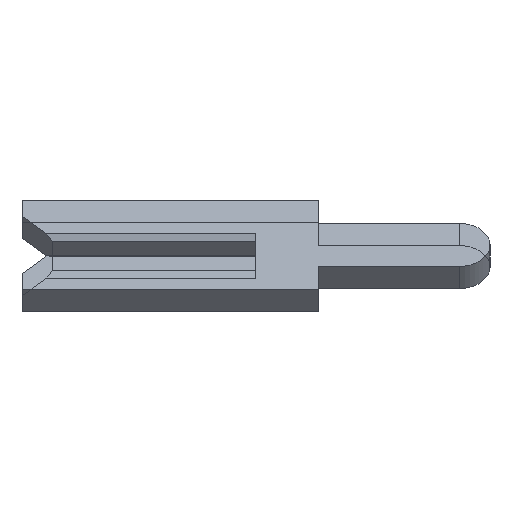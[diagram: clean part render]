
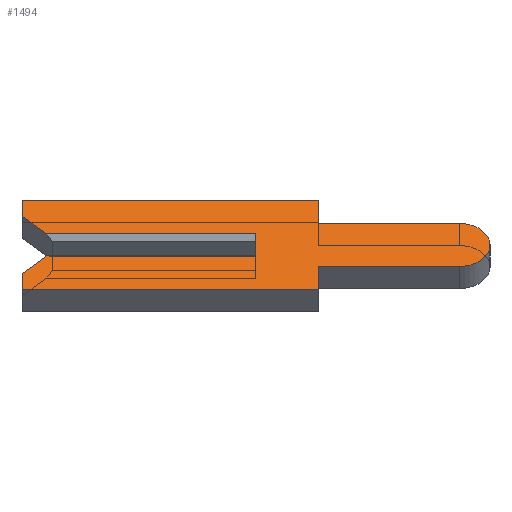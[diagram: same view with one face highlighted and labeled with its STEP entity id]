
A CAD part, left-side view. The second image highlights one B-rep face of the part: STEP entity #1494.
In plain terms, the highlighted face is planar.
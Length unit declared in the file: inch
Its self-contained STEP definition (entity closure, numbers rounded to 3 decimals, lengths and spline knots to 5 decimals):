
#64 = VECTOR ( 'NONE', #1680, 39.37008 ) ;
#102 = CARTESIAN_POINT ( 'NONE',  ( -0.01, -0.1305, 0. ) ) ;
#106 = EDGE_CURVE ( 'NONE', #2117, #2384, #666, .T. ) ;
#193 = CARTESIAN_POINT ( 'NONE',  ( -0.01, 0.1305, -0.0065 ) ) ;
#197 = DIRECTION ( 'NONE',  ( 0., -1., 0. ) ) ;
#211 = DIRECTION ( 'NONE',  ( 0., 0., 1. ) ) ;
#248 = CARTESIAN_POINT ( 'NONE',  ( -0.01, 0.1305, 0.0065 ) ) ;
#283 = EDGE_CURVE ( 'NONE', #1626, #2117, #3240, .T. ) ;
#307 = EDGE_CURVE ( 'NONE', #2683, #2259, #496, .T. ) ;
#316 = AXIS2_PLACEMENT_3D ( 'NONE', #2590, #2842, #1253 ) ;
#362 = LINE ( 'NONE', #2510, #64 ) ;
#367 = DIRECTION ( 'NONE',  ( 0., -1., 0. ) ) ;
#412 = CARTESIAN_POINT ( 'NONE',  ( -0.01, 0.15, 0.026 ) ) ;
#459 = EDGE_CURVE ( 'NONE', #3338, #1836, #2913, .T. ) ;
#496 = LINE ( 'NONE', #1539, #2457 ) ;
#546 = EDGE_CURVE ( 'NONE', #2349, #2683, #1411, .T. ) ;
#647 = ORIENTED_EDGE ( 'NONE', *, *, #3084, .F. ) ;
#666 = LINE ( 'NONE', #770, #1585 ) ;
#696 = CARTESIAN_POINT ( 'NONE',  ( -0.01, -0.04, 0.0195 ) ) ;
#734 = VERTEX_POINT ( 'NONE', #1851 ) ;
#758 = EDGE_CURVE ( 'NONE', #2086, #2349, #2542, .T. ) ;
#770 = CARTESIAN_POINT ( 'NONE',  ( -0.01, 0.15, 0.026 ) ) ;
#792 = LINE ( 'NONE', #860, #1212 ) ;
#850 = DIRECTION ( 'NONE',  ( 0., 0., -1. ) ) ;
#860 = CARTESIAN_POINT ( 'NONE',  ( -0.01, 0.15, 0.01 ) ) ;
#920 = DIRECTION ( 'NONE',  ( 0., 0., -1. ) ) ;
#921 = LINE ( 'NONE', #3278, #3073 ) ;
#983 = EDGE_CURVE ( 'NONE', #2969, #1661, #1864, .T. ) ;
#994 = CARTESIAN_POINT ( 'NONE',  ( -0.01, -0.04, -0.04 ) ) ;
#1008 = ORIENTED_EDGE ( 'NONE', *, *, #2205, .F. ) ;
#1032 = VECTOR ( 'NONE', #367, 39.37008 ) ;
#1094 = ORIENTED_EDGE ( 'NONE', *, *, #459, .F. ) ;
#1099 = AXIS2_PLACEMENT_3D ( 'NONE', #102, #3271, #850 ) ;
#1111 = DIRECTION ( 'NONE',  ( 0., -1., 0. ) ) ;
#1140 = CARTESIAN_POINT ( 'NONE',  ( -0.01, 0., 0.01 ) ) ;
#1164 = EDGE_CURVE ( 'NONE', #1661, #1456, #921, .T. ) ;
#1212 = VECTOR ( 'NONE', #1111, 39.37008 ) ;
#1213 = CARTESIAN_POINT ( 'NONE',  ( -0.01, 0.15, -0.04 ) ) ;
#1216 = ORIENTED_EDGE ( 'NONE', *, *, #2727, .F. ) ;
#1253 = DIRECTION ( 'NONE',  ( 0., 0., -1. ) ) ;
#1291 = FACE_OUTER_BOUND ( 'NONE', #2130, .T. ) ;
#1396 = DIRECTION ( 'NONE',  ( 0., 0., 1. ) ) ;
#1411 = LINE ( 'NONE', #3182, #2415 ) ;
#1428 = DIRECTION ( 'NONE',  ( 0., 0., 1. ) ) ;
#1456 = VERTEX_POINT ( 'NONE', #1140 ) ;
#1494 = ADVANCED_FACE ( 'NONE', ( #1291 ), #2448, .F. ) ;
#1495 = ORIENTED_EDGE ( 'NONE', *, *, #1522, .T. ) ;
#1522 = EDGE_CURVE ( 'NONE', #1626, #1456, #792, .T. ) ;
#1539 = CARTESIAN_POINT ( 'NONE',  ( -0.01, 0.15, -0.04 ) ) ;
#1585 = VECTOR ( 'NONE', #211, 39.37008 ) ;
#1626 = VERTEX_POINT ( 'NONE', #2989 ) ;
#1661 = VERTEX_POINT ( 'NONE', #3243 ) ;
#1680 = DIRECTION ( 'NONE',  ( 0., -1., 0. ) ) ;
#1752 = CARTESIAN_POINT ( 'NONE',  ( -0.01, 0.134, -0.01 ) ) ;
#1791 = LINE ( 'NONE', #1961, #2630 ) ;
#1792 = ORIENTED_EDGE ( 'NONE', *, *, #983, .F. ) ;
#1817 = VECTOR ( 'NONE', #2419, 39.37008 ) ;
#1831 = VECTOR ( 'NONE', #1428, 39.37008 ) ;
#1836 = VERTEX_POINT ( 'NONE', #3004 ) ;
#1851 = CARTESIAN_POINT ( 'NONE',  ( -0.01, 0.15, -0.026 ) ) ;
#1861 = ORIENTED_EDGE ( 'NONE', *, *, #546, .F. ) ;
#1864 = LINE ( 'NONE', #2706, #1032 ) ;
#1924 = LINE ( 'NONE', #193, #3014 ) ;
#1961 = CARTESIAN_POINT ( 'NONE',  ( -0.01, -0.04, 0.04 ) ) ;
#1968 = ORIENTED_EDGE ( 'NONE', *, *, #106, .F. ) ;
#2036 = ORIENTED_EDGE ( 'NONE', *, *, #283, .F. ) ;
#2038 = DIRECTION ( 'NONE',  ( 0., -0.707, 0.707 ) ) ;
#2056 = VERTEX_POINT ( 'NONE', #3292 ) ;
#2078 = CARTESIAN_POINT ( 'NONE',  ( -0.01, -0.04, 0.0195 ) ) ;
#2086 = VERTEX_POINT ( 'NONE', #2548 ) ;
#2117 = VERTEX_POINT ( 'NONE', #412 ) ;
#2130 = EDGE_LOOP ( 'NONE', ( #1495, #2407, #1792, #647, #1216, #2881, #1861, #2634, #2802, #1094, #2217, #1008, #1968, #2036 ) ) ;
#2203 = VECTOR ( 'NONE', #197, 39.37008 ) ;
#2205 = EDGE_CURVE ( 'NONE', #2384, #2056, #362, .T. ) ;
#2217 = ORIENTED_EDGE ( 'NONE', *, *, #2230, .F. ) ;
#2230 = EDGE_CURVE ( 'NONE', #2056, #3338, #1791, .T. ) ;
#2236 = CARTESIAN_POINT ( 'NONE',  ( -0.01, 0.15, -0.026 ) ) ;
#2259 = VERTEX_POINT ( 'NONE', #1213 ) ;
#2320 = DIRECTION ( 'NONE',  ( 0., 0.707, 0.707 ) ) ;
#2349 = VERTEX_POINT ( 'NONE', #3310 ) ;
#2384 = VERTEX_POINT ( 'NONE', #3036 ) ;
#2394 = DIRECTION ( 'NONE',  ( 0., 0., -1. ) ) ;
#2407 = ORIENTED_EDGE ( 'NONE', *, *, #1164, .F. ) ;
#2415 = VECTOR ( 'NONE', #2394, 39.37008 ) ;
#2419 = DIRECTION ( 'NONE',  ( 0., 1., 0. ) ) ;
#2448 = PLANE ( 'NONE',  #1099 ) ;
#2457 = VECTOR ( 'NONE', #3137, 39.37008 ) ;
#2510 = CARTESIAN_POINT ( 'NONE',  ( -0.01, 0.15, 0.04 ) ) ;
#2542 = LINE ( 'NONE', #2671, #1817 ) ;
#2548 = CARTESIAN_POINT ( 'NONE',  ( -0.01, -0.1305, -0.0195 ) ) ;
#2555 = LINE ( 'NONE', #2236, #1831 ) ;
#2590 = CARTESIAN_POINT ( 'NONE',  ( -0.01, -0.1305, 0. ) ) ;
#2630 = VECTOR ( 'NONE', #920, 39.37008 ) ;
#2634 = ORIENTED_EDGE ( 'NONE', *, *, #758, .F. ) ;
#2671 = CARTESIAN_POINT ( 'NONE',  ( -0.01, -0.04, -0.0195 ) ) ;
#2683 = VERTEX_POINT ( 'NONE', #994 ) ;
#2706 = CARTESIAN_POINT ( 'NONE',  ( -0.01, -0.1305, -0.01 ) ) ;
#2727 = EDGE_CURVE ( 'NONE', #2259, #734, #2555, .T. ) ;
#2796 = CIRCLE ( 'NONE', #316, 0.0195 ) ;
#2802 = ORIENTED_EDGE ( 'NONE', *, *, #3173, .F. ) ;
#2842 = DIRECTION ( 'NONE',  ( 1., 0., 0. ) ) ;
#2881 = ORIENTED_EDGE ( 'NONE', *, *, #307, .F. ) ;
#2913 = LINE ( 'NONE', #2078, #2203 ) ;
#2969 = VERTEX_POINT ( 'NONE', #1752 ) ;
#2989 = CARTESIAN_POINT ( 'NONE',  ( -0.01, 0.134, 0.01 ) ) ;
#3004 = CARTESIAN_POINT ( 'NONE',  ( -0.01, -0.1305, 0.0195 ) ) ;
#3014 = VECTOR ( 'NONE', #2038, 39.37008 ) ;
#3036 = CARTESIAN_POINT ( 'NONE',  ( -0.01, 0.15, 0.04 ) ) ;
#3073 = VECTOR ( 'NONE', #1396, 39.37008 ) ;
#3084 = EDGE_CURVE ( 'NONE', #734, #2969, #1924, .T. ) ;
#3137 = DIRECTION ( 'NONE',  ( 0., 1., 0. ) ) ;
#3150 = VECTOR ( 'NONE', #2320, 39.37008 ) ;
#3173 = EDGE_CURVE ( 'NONE', #1836, #2086, #2796, .T. ) ;
#3182 = CARTESIAN_POINT ( 'NONE',  ( -0.01, -0.04, -0.04 ) ) ;
#3240 = LINE ( 'NONE', #248, #3150 ) ;
#3243 = CARTESIAN_POINT ( 'NONE',  ( -0.01, 0., -0.01 ) ) ;
#3271 = DIRECTION ( 'NONE',  ( 1., 0., 0. ) ) ;
#3278 = CARTESIAN_POINT ( 'NONE',  ( -0.01, 0., 0.0065 ) ) ;
#3292 = CARTESIAN_POINT ( 'NONE',  ( -0.01, -0.04, 0.04 ) ) ;
#3310 = CARTESIAN_POINT ( 'NONE',  ( -0.01, -0.04, -0.0195 ) ) ;
#3338 = VERTEX_POINT ( 'NONE', #696 ) ;
